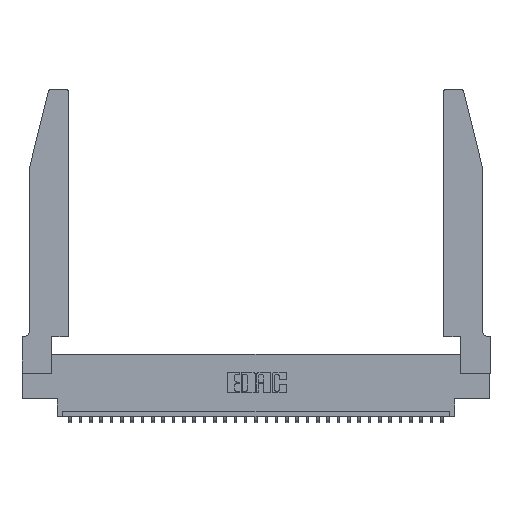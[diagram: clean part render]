
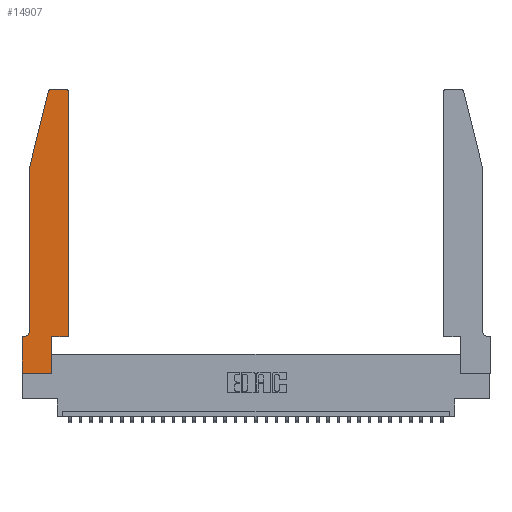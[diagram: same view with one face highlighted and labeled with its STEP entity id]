
A CAD part, top view. The second image highlights one B-rep face of the part: STEP entity #14907.
In plain terms, the highlighted planar face has unit normal (0, 0, 1).
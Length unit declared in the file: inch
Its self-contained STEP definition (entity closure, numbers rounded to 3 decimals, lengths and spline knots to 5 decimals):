
#92 = CARTESIAN_POINT ( 'NONE',  ( 0., 0.35, 0.37 ) ) ;
#310 = EDGE_LOOP ( 'NONE', ( #30491, #20595, #10932, #5381, #15784, #12887, #15595, #346, #29148, #5578, #6184, #31319 ) ) ;
#346 = ORIENTED_EDGE ( 'NONE', *, *, #5235, .T. ) ;
#991 = CARTESIAN_POINT ( 'NONE',  ( 0.2865, 0.35, 0.37 ) ) ;
#1334 = EDGE_CURVE ( 'NONE', #11081, #21697, #32651, .T. ) ;
#1735 = FACE_OUTER_BOUND ( 'NONE', #310, .T. ) ;
#2241 = CARTESIAN_POINT ( 'NONE',  ( 0.2865, 0.35, 0.37 ) ) ;
#2454 = CARTESIAN_POINT ( 'NONE',  ( 0.4505, 0.35, 0.37 ) ) ;
#3790 = CARTESIAN_POINT ( 'NONE',  ( 0.4505, 2.72, 0.37 ) ) ;
#3818 = CARTESIAN_POINT ( 'NONE',  ( 0.0055, 0.42, 0.37 ) ) ;
#4001 = CARTESIAN_POINT ( 'NONE',  ( 0.25487, 2.72718, 0.37 ) ) ;
#4374 = LINE ( 'NONE', #8508, #14444 ) ;
#4391 = VERTEX_POINT ( 'NONE', #4001 ) ;
#5235 = EDGE_CURVE ( 'NONE', #19030, #16958, #22329, .T. ) ;
#5381 = ORIENTED_EDGE ( 'NONE', *, *, #11213, .T. ) ;
#5577 = VERTEX_POINT ( 'NONE', #7200 ) ;
#5578 = ORIENTED_EDGE ( 'NONE', *, *, #12190, .T. ) ;
#6109 = DIRECTION ( 'NONE',  ( 1., 0., 0. ) ) ;
#6184 = ORIENTED_EDGE ( 'NONE', *, *, #1334, .T. ) ;
#6309 = DIRECTION ( 'NONE',  ( 0., 1., 0. ) ) ;
#6431 = DIRECTION ( 'NONE',  ( 0., 0., -1. ) ) ;
#6696 = VERTEX_POINT ( 'NONE', #27129 ) ;
#7200 = CARTESIAN_POINT ( 'NONE',  ( 0.284, 2.75, 0.37 ) ) ;
#7235 = AXIS2_PLACEMENT_3D ( 'NONE', #31822, #18877, #6109 ) ;
#7488 = EDGE_CURVE ( 'NONE', #21697, #13561, #25042, .T. ) ;
#7492 = AXIS2_PLACEMENT_3D ( 'NONE', #92, #31154, #18100 ) ;
#8353 = CARTESIAN_POINT ( 'NONE',  ( 0., 0., 0.37 ) ) ;
#8508 = CARTESIAN_POINT ( 'NONE',  ( 0.0755, 2., 0.37 ) ) ;
#9011 = DIRECTION ( 'NONE',  ( -1., 0., 0. ) ) ;
#9946 = VECTOR ( 'NONE', #31363, 39.37008 ) ;
#10090 = DIRECTION ( 'NONE',  ( 1., 0., 0. ) ) ;
#10148 = AXIS2_PLACEMENT_3D ( 'NONE', #25585, #25147, #27867 ) ;
#10932 = ORIENTED_EDGE ( 'NONE', *, *, #22517, .T. ) ;
#11081 = VERTEX_POINT ( 'NONE', #18788 ) ;
#11212 = AXIS2_PLACEMENT_3D ( 'NONE', #3818, #6431, #9011 ) ;
#11213 = EDGE_CURVE ( 'NONE', #25656, #23803, #4374, .T. ) ;
#11290 = CIRCLE ( 'NONE', #7235, 0.03 ) ;
#11612 = DIRECTION ( 'NONE',  ( 0., -1., 0. ) ) ;
#12190 = EDGE_CURVE ( 'NONE', #13016, #11081, #13517, .T. ) ;
#12887 = ORIENTED_EDGE ( 'NONE', *, *, #21059, .T. ) ;
#12946 = CARTESIAN_POINT ( 'NONE',  ( 0., 0., 0.37 ) ) ;
#13016 = VERTEX_POINT ( 'NONE', #2241 ) ;
#13517 = LINE ( 'NONE', #14796, #14348 ) ;
#13561 = VERTEX_POINT ( 'NONE', #30700 ) ;
#14348 = VECTOR ( 'NONE', #10090, 39.37008 ) ;
#14444 = VECTOR ( 'NONE', #19064, 39.37008 ) ;
#14796 = CARTESIAN_POINT ( 'NONE',  ( 0.4505, 0.35, 0.37 ) ) ;
#14851 = DIRECTION ( 'NONE',  ( 1., 0., 0. ) ) ;
#14856 = LINE ( 'NONE', #27793, #31414 ) ;
#14907 = ADVANCED_FACE ( 'NONE', ( #1735 ), #28454, .T. ) ;
#14991 = DIRECTION ( 'NONE',  ( -1., 0., 0. ) ) ;
#15151 = VECTOR ( 'NONE', #14991, 39.37008 ) ;
#15273 = DIRECTION ( 'NONE',  ( 0., 1., 0. ) ) ;
#15595 = ORIENTED_EDGE ( 'NONE', *, *, #19667, .T. ) ;
#15784 = ORIENTED_EDGE ( 'NONE', *, *, #22059, .T. ) ;
#16221 = CARTESIAN_POINT ( 'NONE',  ( 0.0755, 2., 0.37 ) ) ;
#16958 = VERTEX_POINT ( 'NONE', #24713 ) ;
#18100 = DIRECTION ( 'NONE',  ( 1., 0., 0. ) ) ;
#18357 = CIRCLE ( 'NONE', #11212, 0.07 ) ;
#18788 = CARTESIAN_POINT ( 'NONE',  ( 0.4505, 0.35, 0.37 ) ) ;
#18877 = DIRECTION ( 'NONE',  ( 0., 0., 1. ) ) ;
#19030 = VERTEX_POINT ( 'NONE', #12946 ) ;
#19064 = DIRECTION ( 'NONE',  ( 0., -1., 0. ) ) ;
#19532 = CARTESIAN_POINT ( 'NONE',  ( 0.0755, 0.42, 0.37 ) ) ;
#19667 = EDGE_CURVE ( 'NONE', #21264, #19030, #29214, .T. ) ;
#20166 = EDGE_CURVE ( 'NONE', #16958, #13016, #24619, .T. ) ;
#20595 = ORIENTED_EDGE ( 'NONE', *, *, #24209, .T. ) ;
#21059 = EDGE_CURVE ( 'NONE', #6696, #21264, #14856, .T. ) ;
#21264 = VERTEX_POINT ( 'NONE', #29215 ) ;
#21697 = VERTEX_POINT ( 'NONE', #3790 ) ;
#22059 = EDGE_CURVE ( 'NONE', #23803, #6696, #18357, .T. ) ;
#22329 = LINE ( 'NONE', #24792, #28047 ) ;
#22335 = VECTOR ( 'NONE', #11612, 39.37008 ) ;
#22517 = EDGE_CURVE ( 'NONE', #4391, #25656, #26853, .T. ) ;
#22562 = EDGE_CURVE ( 'NONE', #13561, #5577, #25698, .T. ) ;
#23803 = VERTEX_POINT ( 'NONE', #19532 ) ;
#24209 = EDGE_CURVE ( 'NONE', #5577, #4391, #11290, .T. ) ;
#24619 = LINE ( 'NONE', #991, #28672 ) ;
#24713 = CARTESIAN_POINT ( 'NONE',  ( 0.2865, 0., 0.37 ) ) ;
#24792 = CARTESIAN_POINT ( 'NONE',  ( 0., 0., 0.37 ) ) ;
#25042 = CIRCLE ( 'NONE', #10148, 0.03 ) ;
#25147 = DIRECTION ( 'NONE',  ( 0., 0., 1. ) ) ;
#25585 = CARTESIAN_POINT ( 'NONE',  ( 0.4205, 2.72, 0.37 ) ) ;
#25656 = VERTEX_POINT ( 'NONE', #16221 ) ;
#25698 = LINE ( 'NONE', #32880, #15151 ) ;
#26853 = LINE ( 'NONE', #29659, #9946 ) ;
#27129 = CARTESIAN_POINT ( 'NONE',  ( 0.0055, 0.35, 0.37 ) ) ;
#27556 = DIRECTION ( 'NONE',  ( -1., 0., 0. ) ) ;
#27793 = CARTESIAN_POINT ( 'NONE',  ( 0.0755, 0.35, 0.37 ) ) ;
#27867 = DIRECTION ( 'NONE',  ( 1., 0., 0. ) ) ;
#28047 = VECTOR ( 'NONE', #14851, 39.37008 ) ;
#28454 = PLANE ( 'NONE',  #7492 ) ;
#28672 = VECTOR ( 'NONE', #6309, 39.37008 ) ;
#29148 = ORIENTED_EDGE ( 'NONE', *, *, #20166, .T. ) ;
#29214 = LINE ( 'NONE', #8353, #22335 ) ;
#29215 = CARTESIAN_POINT ( 'NONE',  ( 0., 0.35, 0.37 ) ) ;
#29659 = CARTESIAN_POINT ( 'NONE',  ( 0.0755, 2., 0.37 ) ) ;
#30491 = ORIENTED_EDGE ( 'NONE', *, *, #22562, .T. ) ;
#30700 = CARTESIAN_POINT ( 'NONE',  ( 0.4205, 2.75, 0.37 ) ) ;
#31154 = DIRECTION ( 'NONE',  ( 0., 0., 1. ) ) ;
#31319 = ORIENTED_EDGE ( 'NONE', *, *, #7488, .T. ) ;
#31363 = DIRECTION ( 'NONE',  ( -0.239, -0.971, 0. ) ) ;
#31414 = VECTOR ( 'NONE', #27556, 39.37008 ) ;
#31799 = VECTOR ( 'NONE', #15273, 39.37008 ) ;
#31822 = CARTESIAN_POINT ( 'NONE',  ( 0.284, 2.72, 0.37 ) ) ;
#32651 = LINE ( 'NONE', #2454, #31799 ) ;
#32880 = CARTESIAN_POINT ( 'NONE',  ( 0.2605, 2.75, 0.37 ) ) ;
